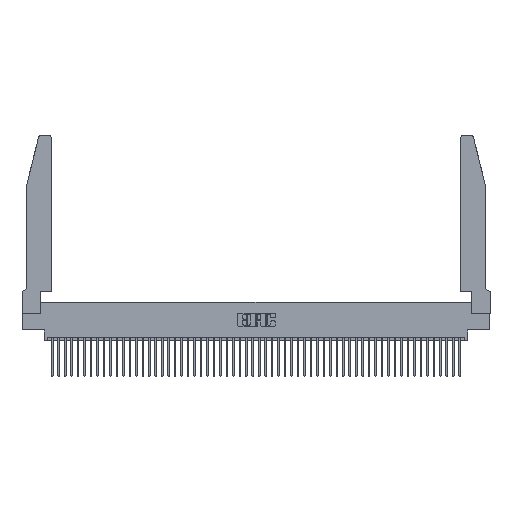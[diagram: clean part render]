
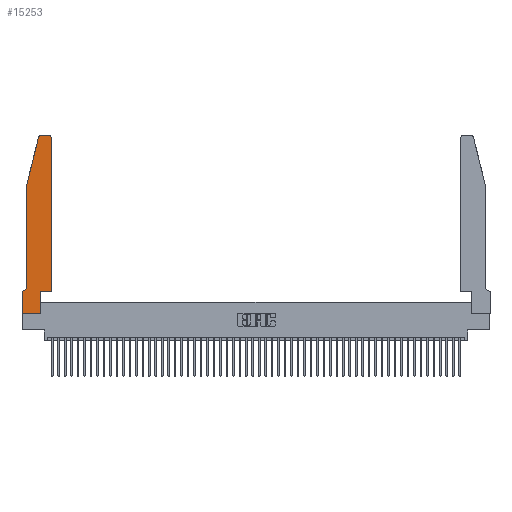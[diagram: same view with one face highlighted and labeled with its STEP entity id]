
A CAD part, top view. The second image highlights one B-rep face of the part: STEP entity #15253.
In plain terms, the highlighted planar face has unit normal (0, 0, 1).
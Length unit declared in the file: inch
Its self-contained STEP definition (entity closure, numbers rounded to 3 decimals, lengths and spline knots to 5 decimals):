
#920 = VERTEX_POINT ( 'NONE', #51786 ) ;
#1158 = VECTOR ( 'NONE', #36133, 39.37008 ) ;
#1414 = CARTESIAN_POINT ( 'NONE',  ( 0.2865, 0., 0.37 ) ) ;
#1999 = VECTOR ( 'NONE', #17190, 39.37008 ) ;
#2759 = CARTESIAN_POINT ( 'NONE',  ( 0.4205, 2.72, 0.37 ) ) ;
#3172 = EDGE_CURVE ( 'NONE', #25665, #21749, #32441, .T. ) ;
#3735 = ORIENTED_EDGE ( 'NONE', *, *, #18640, .T. ) ;
#3768 = DIRECTION ( 'NONE',  ( -1., 0., 0. ) ) ;
#4591 = EDGE_CURVE ( 'NONE', #27214, #25665, #10034, .T. ) ;
#4652 = CARTESIAN_POINT ( 'NONE',  ( 0.0755, 2., 0.37 ) ) ;
#6304 = LINE ( 'NONE', #25836, #51099 ) ;
#6647 = CARTESIAN_POINT ( 'NONE',  ( 0.284, 2.72, 0.37 ) ) ;
#6868 = ORIENTED_EDGE ( 'NONE', *, *, #45964, .T. ) ;
#6922 = ORIENTED_EDGE ( 'NONE', *, *, #27965, .T. ) ;
#7173 = DIRECTION ( 'NONE',  ( 1., 0., 0. ) ) ;
#7727 = AXIS2_PLACEMENT_3D ( 'NONE', #6647, #23222, #7173 ) ;
#8039 = CARTESIAN_POINT ( 'NONE',  ( 0.0055, 0.42, 0.37 ) ) ;
#8203 = DIRECTION ( 'NONE',  ( 0., 0., 1. ) ) ;
#10034 = LINE ( 'NONE', #48034, #34054 ) ;
#10966 = LINE ( 'NONE', #43232, #29974 ) ;
#11921 = EDGE_CURVE ( 'NONE', #34761, #35281, #6304, .T. ) ;
#12264 = AXIS2_PLACEMENT_3D ( 'NONE', #24602, #8203, #16496 ) ;
#12592 = VERTEX_POINT ( 'NONE', #1414 ) ;
#12982 = EDGE_CURVE ( 'NONE', #40129, #34761, #27720, .T. ) ;
#14089 = CARTESIAN_POINT ( 'NONE',  ( 0.0055, 0.35, 0.37 ) ) ;
#14352 = ORIENTED_EDGE ( 'NONE', *, *, #21022, .T. ) ;
#14428 = VERTEX_POINT ( 'NONE', #39612 ) ;
#14660 = VERTEX_POINT ( 'NONE', #16197 ) ;
#14718 = CARTESIAN_POINT ( 'NONE',  ( 0.4505, 0.35, 0.37 ) ) ;
#14748 = DIRECTION ( 'NONE',  ( 1., 0., 0. ) ) ;
#15253 = ADVANCED_FACE ( 'NONE', ( #47660 ), #44317, .T. ) ;
#15972 = CIRCLE ( 'NONE', #26682, 0.07 ) ;
#16197 = CARTESIAN_POINT ( 'NONE',  ( 0.25487, 2.72718, 0.37 ) ) ;
#16496 = DIRECTION ( 'NONE',  ( 1., 0., 0. ) ) ;
#17190 = DIRECTION ( 'NONE',  ( -0.239, -0.971, 0. ) ) ;
#17900 = CIRCLE ( 'NONE', #20209, 0.03 ) ;
#18640 = EDGE_CURVE ( 'NONE', #47333, #920, #36896, .T. ) ;
#20209 = AXIS2_PLACEMENT_3D ( 'NONE', #2759, #39232, #14748 ) ;
#20412 = CARTESIAN_POINT ( 'NONE',  ( 0.2605, 2.75, 0.37 ) ) ;
#20536 = DIRECTION ( 'NONE',  ( -1., 0., 0. ) ) ;
#20737 = EDGE_CURVE ( 'NONE', #35281, #14428, #17900, .T. ) ;
#21022 = EDGE_CURVE ( 'NONE', #920, #27214, #15972, .T. ) ;
#21749 = VERTEX_POINT ( 'NONE', #41707 ) ;
#23222 = DIRECTION ( 'NONE',  ( 0., 0., 1. ) ) ;
#24602 = CARTESIAN_POINT ( 'NONE',  ( 0., 0.35, 0.37 ) ) ;
#24829 = CARTESIAN_POINT ( 'NONE',  ( 0.4505, 0.35, 0.37 ) ) ;
#25665 = VERTEX_POINT ( 'NONE', #44910 ) ;
#25836 = CARTESIAN_POINT ( 'NONE',  ( 0.4505, 0.35, 0.37 ) ) ;
#25963 = CARTESIAN_POINT ( 'NONE',  ( 0.284, 2.75, 0.37 ) ) ;
#26074 = ORIENTED_EDGE ( 'NONE', *, *, #12982, .T. ) ;
#26682 = AXIS2_PLACEMENT_3D ( 'NONE', #8039, #40442, #20536 ) ;
#26935 = DIRECTION ( 'NONE',  ( 1., 0., 0. ) ) ;
#27214 = VERTEX_POINT ( 'NONE', #14089 ) ;
#27720 = LINE ( 'NONE', #24829, #1158 ) ;
#27965 = EDGE_CURVE ( 'NONE', #21749, #12592, #10966, .T. ) ;
#29036 = ORIENTED_EDGE ( 'NONE', *, *, #20737, .T. ) ;
#29095 = ORIENTED_EDGE ( 'NONE', *, *, #44948, .T. ) ;
#29974 = VECTOR ( 'NONE', #26935, 39.37008 ) ;
#30575 = CARTESIAN_POINT ( 'NONE',  ( 0.0755, 2., 0.37 ) ) ;
#31302 = DIRECTION ( 'NONE',  ( 0., -1., 0. ) ) ;
#31423 = ORIENTED_EDGE ( 'NONE', *, *, #33802, .T. ) ;
#32351 = LINE ( 'NONE', #49703, #49334 ) ;
#32441 = LINE ( 'NONE', #39498, #47508 ) ;
#32956 = LINE ( 'NONE', #4652, #1999 ) ;
#33461 = ORIENTED_EDGE ( 'NONE', *, *, #38320, .T. ) ;
#33802 = EDGE_CURVE ( 'NONE', #14660, #47333, #32956, .T. ) ;
#34054 = VECTOR ( 'NONE', #3768, 39.37008 ) ;
#34112 = DIRECTION ( 'NONE',  ( 0., 1., 0. ) ) ;
#34761 = VERTEX_POINT ( 'NONE', #14718 ) ;
#34973 = CIRCLE ( 'NONE', #7727, 0.03 ) ;
#35152 = DIRECTION ( 'NONE',  ( 0., -1., 0. ) ) ;
#35281 = VERTEX_POINT ( 'NONE', #44824 ) ;
#36133 = DIRECTION ( 'NONE',  ( 1., 0., 0. ) ) ;
#36896 = LINE ( 'NONE', #51266, #38140 ) ;
#37482 = VECTOR ( 'NONE', #48623, 39.37008 ) ;
#38140 = VECTOR ( 'NONE', #31302, 39.37008 ) ;
#38320 = EDGE_CURVE ( 'NONE', #14428, #45927, #49465, .T. ) ;
#38486 = ORIENTED_EDGE ( 'NONE', *, *, #11921, .T. ) ;
#38946 = DIRECTION ( 'NONE',  ( 0., 1., 0. ) ) ;
#39096 = CARTESIAN_POINT ( 'NONE',  ( 0.2865, 0.35, 0.37 ) ) ;
#39232 = DIRECTION ( 'NONE',  ( 0., 0., 1. ) ) ;
#39498 = CARTESIAN_POINT ( 'NONE',  ( 0., 0., 0.37 ) ) ;
#39612 = CARTESIAN_POINT ( 'NONE',  ( 0.4205, 2.75, 0.37 ) ) ;
#40129 = VERTEX_POINT ( 'NONE', #39096 ) ;
#40442 = DIRECTION ( 'NONE',  ( 0., 0., -1. ) ) ;
#41707 = CARTESIAN_POINT ( 'NONE',  ( 0., 0., 0.37 ) ) ;
#43232 = CARTESIAN_POINT ( 'NONE',  ( 0., 0., 0.37 ) ) ;
#43369 = ORIENTED_EDGE ( 'NONE', *, *, #4591, .T. ) ;
#44317 = PLANE ( 'NONE',  #12264 ) ;
#44824 = CARTESIAN_POINT ( 'NONE',  ( 0.4505, 2.72, 0.37 ) ) ;
#44910 = CARTESIAN_POINT ( 'NONE',  ( 0., 0.35, 0.37 ) ) ;
#44948 = EDGE_CURVE ( 'NONE', #45927, #14660, #34973, .T. ) ;
#45844 = ORIENTED_EDGE ( 'NONE', *, *, #3172, .T. ) ;
#45927 = VERTEX_POINT ( 'NONE', #25963 ) ;
#45964 = EDGE_CURVE ( 'NONE', #12592, #40129, #32351, .T. ) ;
#47333 = VERTEX_POINT ( 'NONE', #30575 ) ;
#47508 = VECTOR ( 'NONE', #35152, 39.37008 ) ;
#47660 = FACE_OUTER_BOUND ( 'NONE', #50950, .T. ) ;
#48034 = CARTESIAN_POINT ( 'NONE',  ( 0.0755, 0.35, 0.37 ) ) ;
#48623 = DIRECTION ( 'NONE',  ( -1., 0., 0. ) ) ;
#49334 = VECTOR ( 'NONE', #38946, 39.37008 ) ;
#49465 = LINE ( 'NONE', #20412, #37482 ) ;
#49703 = CARTESIAN_POINT ( 'NONE',  ( 0.2865, 0.35, 0.37 ) ) ;
#50950 = EDGE_LOOP ( 'NONE', ( #33461, #29095, #31423, #3735, #14352, #43369, #45844, #6922, #6868, #26074, #38486, #29036 ) ) ;
#51099 = VECTOR ( 'NONE', #34112, 39.37008 ) ;
#51266 = CARTESIAN_POINT ( 'NONE',  ( 0.0755, 2., 0.37 ) ) ;
#51786 = CARTESIAN_POINT ( 'NONE',  ( 0.0755, 0.42, 0.37 ) ) ;
